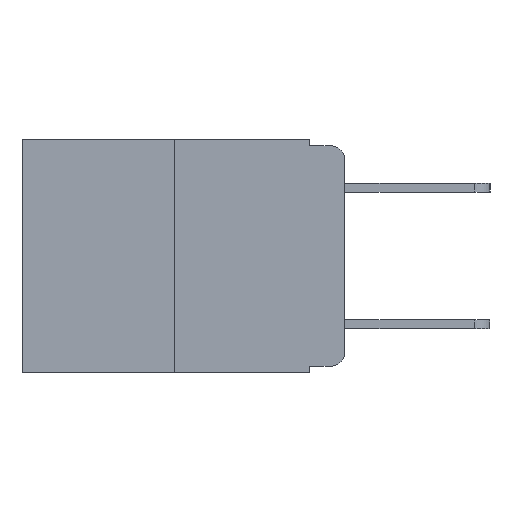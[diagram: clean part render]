
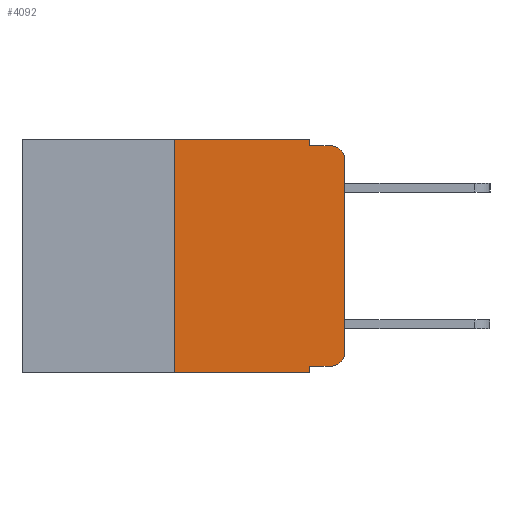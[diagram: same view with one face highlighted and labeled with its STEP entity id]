
A CAD part, left-side view. The second image highlights one B-rep face of the part: STEP entity #4092.
In plain terms, the highlighted planar face has unit normal (-1, 0, 0).
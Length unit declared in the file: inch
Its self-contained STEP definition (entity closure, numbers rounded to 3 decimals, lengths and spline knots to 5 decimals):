
#405 = DIRECTION ( 'NONE',  ( 0., -1., 0. ) ) ;
#479 = LINE ( 'NONE', #13118, #3159 ) ;
#527 = DIRECTION ( 'NONE',  ( 0., -1., 0. ) ) ;
#556 = VERTEX_POINT ( 'NONE', #6775 ) ;
#589 = DIRECTION ( 'NONE',  ( 0., -1., 0. ) ) ;
#630 = CARTESIAN_POINT ( 'NONE',  ( 0., 0.051, 0. ) ) ;
#733 = DIRECTION ( 'NONE',  ( 0., -1., 0. ) ) ;
#751 = VECTOR ( 'NONE', #589, 39.37008 ) ;
#842 = CARTESIAN_POINT ( 'NONE',  ( 0., 0., -0.313 ) ) ;
#1075 = DIRECTION ( 'NONE',  ( 1., 0., 0. ) ) ;
#1241 = EDGE_CURVE ( 'NONE', #1992, #556, #12798, .T. ) ;
#1606 = AXIS2_PLACEMENT_3D ( 'NONE', #6633, #1075, #8725 ) ;
#1776 = ORIENTED_EDGE ( 'NONE', *, *, #3801, .T. ) ;
#1814 = DIRECTION ( 'NONE',  ( 0., 0., -1. ) ) ;
#1945 = ORIENTED_EDGE ( 'NONE', *, *, #1241, .T. ) ;
#1992 = VERTEX_POINT ( 'NONE', #7973 ) ;
#2001 = EDGE_CURVE ( 'NONE', #2927, #1992, #6198, .T. ) ;
#2057 = DIRECTION ( 'NONE',  ( 0., 0., -1. ) ) ;
#2063 = LINE ( 'NONE', #630, #4644 ) ;
#2108 = CARTESIAN_POINT ( 'NONE',  ( 0., 0.051, 0. ) ) ;
#2212 = EDGE_LOOP ( 'NONE', ( #12444, #1945, #13350, #2700, #3049, #8761, #6638, #9689, #9987, #1776 ) ) ;
#2700 = ORIENTED_EDGE ( 'NONE', *, *, #11479, .F. ) ;
#2841 = DIRECTION ( 'NONE',  ( 0., 0., -1. ) ) ;
#2853 = DIRECTION ( 'NONE',  ( -1., 0., 0. ) ) ;
#2927 = VERTEX_POINT ( 'NONE', #842 ) ;
#2941 = CARTESIAN_POINT ( 'NONE',  ( 0., 0.02, -0.03 ) ) ;
#3049 = ORIENTED_EDGE ( 'NONE', *, *, #6942, .F. ) ;
#3159 = VECTOR ( 'NONE', #527, 39.37008 ) ;
#3666 = VECTOR ( 'NONE', #2057, 39.37008 ) ;
#3761 = LINE ( 'NONE', #11236, #751 ) ;
#3801 = EDGE_CURVE ( 'NONE', #4239, #2927, #4529, .T. ) ;
#4092 = ADVANCED_FACE ( 'NONE', ( #8732 ), #13582, .F. ) ;
#4239 = VERTEX_POINT ( 'NONE', #5820 ) ;
#4476 = VERTEX_POINT ( 'NONE', #8037 ) ;
#4529 = CIRCLE ( 'NONE', #8041, 0.02 ) ;
#4644 = VECTOR ( 'NONE', #1814, 39.37008 ) ;
#4957 = VERTEX_POINT ( 'NONE', #5703 ) ;
#5285 = LINE ( 'NONE', #11406, #13080 ) ;
#5703 = CARTESIAN_POINT ( 'NONE',  ( 0., 0.051, 0. ) ) ;
#5704 = LINE ( 'NONE', #7741, #10833 ) ;
#5820 = CARTESIAN_POINT ( 'NONE',  ( 0., 0.02, -0.333 ) ) ;
#6032 = CARTESIAN_POINT ( 'NONE',  ( 0., 0.25, -0.343 ) ) ;
#6066 = VERTEX_POINT ( 'NONE', #7845 ) ;
#6099 = CARTESIAN_POINT ( 'NONE',  ( 0., 0.02, -0.313 ) ) ;
#6198 = LINE ( 'NONE', #9193, #10955 ) ;
#6633 = CARTESIAN_POINT ( 'NONE',  ( 0., 0.473, 0. ) ) ;
#6638 = ORIENTED_EDGE ( 'NONE', *, *, #6836, .T. ) ;
#6734 = EDGE_CURVE ( 'NONE', #6066, #4239, #12930, .T. ) ;
#6775 = CARTESIAN_POINT ( 'NONE',  ( 0., 0.02, -0.01 ) ) ;
#6836 = EDGE_CURVE ( 'NONE', #9033, #9069, #3761, .T. ) ;
#6942 = EDGE_CURVE ( 'NONE', #9307, #4957, #5285, .T. ) ;
#6992 = DIRECTION ( 'NONE',  ( 0., 0., 1. ) ) ;
#7148 = DIRECTION ( 'NONE',  ( 0., 0., -1. ) ) ;
#7450 = EDGE_CURVE ( 'NONE', #6066, #9069, #11941, .T. ) ;
#7741 = CARTESIAN_POINT ( 'NONE',  ( 0., 0.25, 0. ) ) ;
#7845 = CARTESIAN_POINT ( 'NONE',  ( 0., 0.051, -0.333 ) ) ;
#7973 = CARTESIAN_POINT ( 'NONE',  ( 0., 0., -0.03 ) ) ;
#7993 = VECTOR ( 'NONE', #405, 39.37008 ) ;
#8037 = CARTESIAN_POINT ( 'NONE',  ( 0., 0.051, -0.01 ) ) ;
#8041 = AXIS2_PLACEMENT_3D ( 'NONE', #6099, #13102, #7148 ) ;
#8725 = DIRECTION ( 'NONE',  ( 0., 0., -1. ) ) ;
#8732 = FACE_OUTER_BOUND ( 'NONE', #2212, .T. ) ;
#8761 = ORIENTED_EDGE ( 'NONE', *, *, #8832, .F. ) ;
#8832 = EDGE_CURVE ( 'NONE', #9033, #9307, #5704, .T. ) ;
#9033 = VERTEX_POINT ( 'NONE', #6032 ) ;
#9069 = VERTEX_POINT ( 'NONE', #10188 ) ;
#9193 = CARTESIAN_POINT ( 'NONE',  ( 0., 0., 0. ) ) ;
#9307 = VERTEX_POINT ( 'NONE', #13461 ) ;
#9689 = ORIENTED_EDGE ( 'NONE', *, *, #7450, .F. ) ;
#9987 = ORIENTED_EDGE ( 'NONE', *, *, #6734, .T. ) ;
#10188 = CARTESIAN_POINT ( 'NONE',  ( 0., 0.051, -0.343 ) ) ;
#10833 = VECTOR ( 'NONE', #12711, 39.37008 ) ;
#10955 = VECTOR ( 'NONE', #6992, 39.37008 ) ;
#11236 = CARTESIAN_POINT ( 'NONE',  ( 0., 0.473, -0.343 ) ) ;
#11406 = CARTESIAN_POINT ( 'NONE',  ( 0., 0.473, 0. ) ) ;
#11479 = EDGE_CURVE ( 'NONE', #4957, #4476, #2063, .T. ) ;
#11941 = LINE ( 'NONE', #2108, #3666 ) ;
#12122 = EDGE_CURVE ( 'NONE', #4476, #556, #479, .T. ) ;
#12444 = ORIENTED_EDGE ( 'NONE', *, *, #2001, .T. ) ;
#12497 = AXIS2_PLACEMENT_3D ( 'NONE', #2941, #2853, #2841 ) ;
#12711 = DIRECTION ( 'NONE',  ( 0., 0., 1. ) ) ;
#12798 = CIRCLE ( 'NONE', #12497, 0.02 ) ;
#12930 = LINE ( 'NONE', #13015, #7993 ) ;
#13015 = CARTESIAN_POINT ( 'NONE',  ( 0., 0.051, -0.333 ) ) ;
#13080 = VECTOR ( 'NONE', #733, 39.37008 ) ;
#13102 = DIRECTION ( 'NONE',  ( -1., 0., 0. ) ) ;
#13118 = CARTESIAN_POINT ( 'NONE',  ( 0., 0.051, -0.01 ) ) ;
#13350 = ORIENTED_EDGE ( 'NONE', *, *, #12122, .F. ) ;
#13461 = CARTESIAN_POINT ( 'NONE',  ( 0., 0.25, 0. ) ) ;
#13582 = PLANE ( 'NONE',  #1606 ) ;
